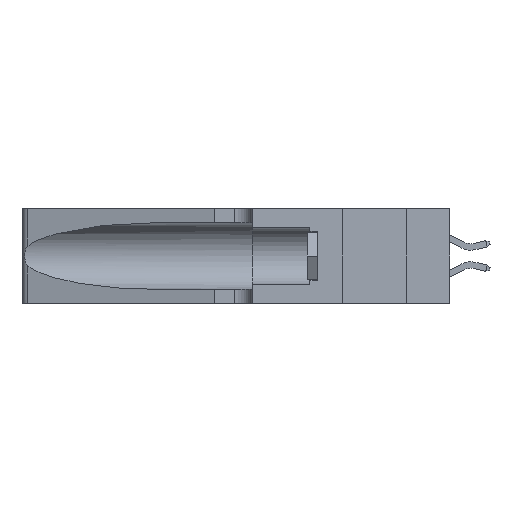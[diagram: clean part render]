
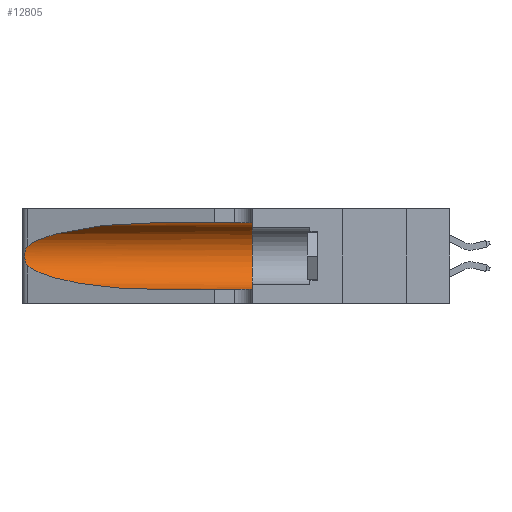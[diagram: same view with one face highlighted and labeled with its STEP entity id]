
A CAD part, left-side view. The second image highlights one B-rep face of the part: STEP entity #12805.
In plain terms, the highlighted cylindrical face has radius 3.308 mm (diameter 6.617 mm), a partial arc.
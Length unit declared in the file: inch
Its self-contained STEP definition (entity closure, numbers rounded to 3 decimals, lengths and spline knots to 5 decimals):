
#390 = CARTESIAN_POINT ( 'NONE',  ( 0.1305, 0.72297, 0.05475 ) ) ;
#875 = LINE ( 'NONE', #19763, #2598 ) ;
#1047 = CARTESIAN_POINT ( 'NONE',  ( 0.25555, 1.22994, 0.2215 ) ) ;
#1124 = CARTESIAN_POINT ( 'NONE',  ( 0.25555, 1.22993, 0.14849 ) ) ;
#1209 =( BOUNDED_CURVE ( )  B_SPLINE_CURVE ( 3, ( #12610, #3520, #17878, #7194 ),
 .UNSPECIFIED., .F., .F. ) 
 B_SPLINE_CURVE_WITH_KNOTS ( ( 4, 4 ),
 ( 1.5708, 2.84003 ),
 .UNSPECIFIED. ) 
 CURVE ( )  GEOMETRIC_REPRESENTATION_ITEM ( )  RATIONAL_B_SPLINE_CURVE ( ( 1., 0.87, 0.87, 1. ) ) 
 REPRESENTATION_ITEM ( '' )  );
#1818 = ORIENTED_EDGE ( 'NONE', *, *, #19577, .T. ) ;
#2159 = CARTESIAN_POINT ( 'NONE',  ( 0.1305, 0.72297, 0.31525 ) ) ;
#2408 = VECTOR ( 'NONE', #10696, 39.37008 ) ;
#2598 = VECTOR ( 'NONE', #3738, 39.37008 ) ;
#2943 = CARTESIAN_POINT ( 'NONE',  ( 0.18966, 0.96281, 0.05475 ) ) ;
#3418 = B_SPLINE_CURVE_WITH_KNOTS ( 'NONE', 3,
 ( #13764, #1047, #15498, #4729, #17275, #6564, #19026, #8395, #20774, #10230, #22526, #12052, #1124, #13838 ),
 .UNSPECIFIED., .F., .F.,
 ( 4, 2, 2, 2, 2, 2, 4 ),
 ( 0., 0.00027, 0.00053, 0.00107, 0.0016, 0.00187, 0.00214 ),
 .UNSPECIFIED. ) ;
#3520 = CARTESIAN_POINT ( 'NONE',  ( 0.18966, 0.96281, 0.31525 ) ) ;
#3738 = DIRECTION ( 'NONE',  ( 0., -1., 0. ) ) ;
#4048 = DIRECTION ( 'NONE',  ( 0., 0., -1. ) ) ;
#4258 = VERTEX_POINT ( 'NONE', #20950 ) ;
#4445 =( BOUNDED_CURVE ( )  B_SPLINE_CURVE ( 3, ( #19010, #12037, #2943, #15563 ),
 .UNSPECIFIED., .F., .T. ) 
 B_SPLINE_CURVE_WITH_KNOTS ( ( 4, 4 ),
 ( 3.44316, 4.71239 ),
 .UNSPECIFIED. ) 
 CURVE ( )  GEOMETRIC_REPRESENTATION_ITEM ( )  RATIONAL_B_SPLINE_CURVE ( ( 1., 0.87, 0.87, 1. ) ) 
 REPRESENTATION_ITEM ( '' )  );
#4556 = DIRECTION ( 'NONE',  ( 0., 1., 0. ) ) ;
#4729 = CARTESIAN_POINT ( 'NONE',  ( 0.25787, 1.23484, 0.2124 ) ) ;
#5249 = VERTEX_POINT ( 'NONE', #2159 ) ;
#5557 = VERTEX_POINT ( 'NONE', #10293 ) ;
#5920 = CARTESIAN_POINT ( 'NONE',  ( 0.1305, 0.35, 0.31525 ) ) ;
#6564 = CARTESIAN_POINT ( 'NONE',  ( 0.26018, 1.23835, 0.19895 ) ) ;
#7022 = CARTESIAN_POINT ( 'NONE',  ( 0.1305, 1.61858, 0.31525 ) ) ;
#7194 = CARTESIAN_POINT ( 'NONE',  ( 0.25487, 1.22718, 0.22369 ) ) ;
#7638 = DIRECTION ( 'NONE',  ( 0., -1., 0. ) ) ;
#8087 = CARTESIAN_POINT ( 'NONE',  ( 0.25487, 1.22718, 0.22369 ) ) ;
#8395 = CARTESIAN_POINT ( 'NONE',  ( 0.26075, 1.23896, 0.178 ) ) ;
#8445 = ORIENTED_EDGE ( 'NONE', *, *, #13712, .T. ) ;
#9477 = CARTESIAN_POINT ( 'NONE',  ( 0.1305, 1.61858, 0.185 ) ) ;
#9968 = AXIS2_PLACEMENT_3D ( 'NONE', #15328, #4556, #17098 ) ;
#9970 = EDGE_CURVE ( 'NONE', #5249, #18650, #16767, .T. ) ;
#10230 = CARTESIAN_POINT ( 'NONE',  ( 0.25856, 1.23593, 0.16098 ) ) ;
#10293 = CARTESIAN_POINT ( 'NONE',  ( 0.1305, 0.35, 0.05475 ) ) ;
#10548 = EDGE_LOOP ( 'NONE', ( #18283, #8445, #20060, #1818, #12246, #17302 ) ) ;
#10696 = DIRECTION ( 'NONE',  ( 0., -1., 0. ) ) ;
#11819 = EDGE_CURVE ( 'NONE', #4258, #12213, #4445, .T. ) ;
#12037 = CARTESIAN_POINT ( 'NONE',  ( 0.2373, 1.15595, 0.08982 ) ) ;
#12052 = CARTESIAN_POINT ( 'NONE',  ( 0.25639, 1.23186, 0.15144 ) ) ;
#12213 = VERTEX_POINT ( 'NONE', #390 ) ;
#12246 = ORIENTED_EDGE ( 'NONE', *, *, #16834, .F. ) ;
#12610 = CARTESIAN_POINT ( 'NONE',  ( 0.1305, 0.72297, 0.31525 ) ) ;
#12805 = ADVANCED_FACE ( 'NONE', ( #23021 ), #20295, .F. ) ;
#13545 = CIRCLE ( 'NONE', #9968, 0.13025 ) ;
#13712 = EDGE_CURVE ( 'NONE', #15415, #4258, #3418, .T. ) ;
#13764 = CARTESIAN_POINT ( 'NONE',  ( 0.25487, 1.22718, 0.22369 ) ) ;
#13838 = CARTESIAN_POINT ( 'NONE',  ( 0.25487, 1.22718, 0.14631 ) ) ;
#15328 = CARTESIAN_POINT ( 'NONE',  ( 0.1305, 0.35, 0.185 ) ) ;
#15415 = VERTEX_POINT ( 'NONE', #8087 ) ;
#15498 = CARTESIAN_POINT ( 'NONE',  ( 0.25639, 1.23184, 0.21858 ) ) ;
#15563 = CARTESIAN_POINT ( 'NONE',  ( 0.1305, 0.72297, 0.05475 ) ) ;
#16767 = LINE ( 'NONE', #7022, #2408 ) ;
#16834 = EDGE_CURVE ( 'NONE', #18650, #5557, #13545, .T. ) ;
#17098 = DIRECTION ( 'NONE',  ( 0., 0., 1. ) ) ;
#17275 = CARTESIAN_POINT ( 'NONE',  ( 0.25854, 1.2359, 0.20912 ) ) ;
#17302 = ORIENTED_EDGE ( 'NONE', *, *, #9970, .F. ) ;
#17878 = CARTESIAN_POINT ( 'NONE',  ( 0.2373, 1.15595, 0.28018 ) ) ;
#18283 = ORIENTED_EDGE ( 'NONE', *, *, #18418, .T. ) ;
#18418 = EDGE_CURVE ( 'NONE', #5249, #15415, #1209, .T. ) ;
#18650 = VERTEX_POINT ( 'NONE', #5920 ) ;
#19010 = CARTESIAN_POINT ( 'NONE',  ( 0.25487, 1.22718, 0.14631 ) ) ;
#19026 = CARTESIAN_POINT ( 'NONE',  ( 0.26075, 1.23896, 0.19203 ) ) ;
#19577 = EDGE_CURVE ( 'NONE', #12213, #5557, #875, .T. ) ;
#19763 = CARTESIAN_POINT ( 'NONE',  ( 0.1305, 1.61858, 0.05475 ) ) ;
#20060 = ORIENTED_EDGE ( 'NONE', *, *, #11819, .T. ) ;
#20295 = CYLINDRICAL_SURFACE ( 'NONE', #21563, 0.13025 ) ;
#20774 = CARTESIAN_POINT ( 'NONE',  ( 0.26017, 1.23833, 0.17102 ) ) ;
#20950 = CARTESIAN_POINT ( 'NONE',  ( 0.25487, 1.22718, 0.14631 ) ) ;
#21563 = AXIS2_PLACEMENT_3D ( 'NONE', #9477, #7638, #4048 ) ;
#22526 = CARTESIAN_POINT ( 'NONE',  ( 0.25789, 1.23486, 0.15765 ) ) ;
#23021 = FACE_OUTER_BOUND ( 'NONE', #10548, .T. ) ;
